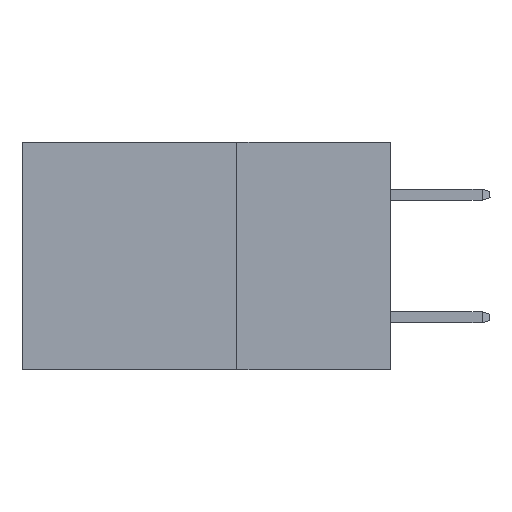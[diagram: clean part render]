
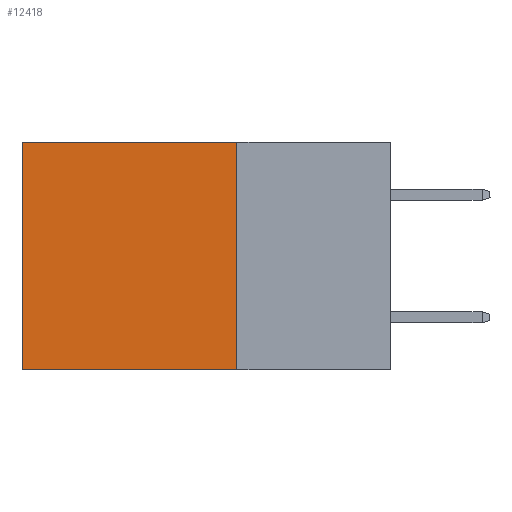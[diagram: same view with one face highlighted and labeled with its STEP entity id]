
A CAD part, left-side view. The second image highlights one B-rep face of the part: STEP entity #12418.
In plain terms, the highlighted planar face has unit normal (-1, 0, 0).
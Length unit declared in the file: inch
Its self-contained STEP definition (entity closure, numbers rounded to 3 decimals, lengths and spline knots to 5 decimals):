
#120 = ORIENTED_EDGE ( 'NONE', *, *, #13641, .F. ) ;
#557 = EDGE_CURVE ( 'NONE', #9670, #3187, #7777, .T. ) ;
#871 = EDGE_CURVE ( 'NONE', #7259, #7469, #4537, .T. ) ;
#1874 = FACE_OUTER_BOUND ( 'NONE', #2642, .T. ) ;
#1922 = CARTESIAN_POINT ( 'NONE',  ( 0.2875, 0.25, -0.37 ) ) ;
#2107 = ORIENTED_EDGE ( 'NONE', *, *, #6444, .T. ) ;
#2642 = EDGE_LOOP ( 'NONE', ( #2107, #12900, #120, #6379 ) ) ;
#2757 = DIRECTION ( 'NONE',  ( 0., 1., 0. ) ) ;
#3071 = DIRECTION ( 'NONE',  ( 0., 0., -1. ) ) ;
#3072 = VECTOR ( 'NONE', #13787, 39.37008 ) ;
#3149 = CARTESIAN_POINT ( 'NONE',  ( 0.2875, 0.6, 0. ) ) ;
#3170 = CARTESIAN_POINT ( 'NONE',  ( 0.2875, 0.25, 0. ) ) ;
#3187 = VERTEX_POINT ( 'NONE', #12374 ) ;
#3828 = VECTOR ( 'NONE', #9761, 39.37008 ) ;
#4186 = VECTOR ( 'NONE', #2757, 39.37008 ) ;
#4537 = LINE ( 'NONE', #3170, #4186 ) ;
#4897 = DIRECTION ( 'NONE',  ( 1., 0., 0. ) ) ;
#5586 = CARTESIAN_POINT ( 'NONE',  ( 0.2875, 0.25, 0. ) ) ;
#5957 = LINE ( 'NONE', #5586, #3072 ) ;
#6084 = CARTESIAN_POINT ( 'NONE',  ( 0.2875, 0.25, -0.37 ) ) ;
#6278 = VECTOR ( 'NONE', #3071, 39.37008 ) ;
#6379 = ORIENTED_EDGE ( 'NONE', *, *, #871, .T. ) ;
#6444 = EDGE_CURVE ( 'NONE', #7469, #3187, #6798, .T. ) ;
#6798 = LINE ( 'NONE', #11131, #6278 ) ;
#7259 = VERTEX_POINT ( 'NONE', #13554 ) ;
#7469 = VERTEX_POINT ( 'NONE', #3149 ) ;
#7777 = LINE ( 'NONE', #6084, #3828 ) ;
#9514 = PLANE ( 'NONE',  #9936 ) ;
#9670 = VERTEX_POINT ( 'NONE', #1922 ) ;
#9761 = DIRECTION ( 'NONE',  ( 0., 1., 0. ) ) ;
#9936 = AXIS2_PLACEMENT_3D ( 'NONE', #11616, #4897, #14061 ) ;
#11131 = CARTESIAN_POINT ( 'NONE',  ( 0.2875, 0.6, 0. ) ) ;
#11616 = CARTESIAN_POINT ( 'NONE',  ( 0.2875, 0.25, 0. ) ) ;
#12374 = CARTESIAN_POINT ( 'NONE',  ( 0.2875, 0.6, -0.37 ) ) ;
#12418 = ADVANCED_FACE ( 'NONE', ( #1874 ), #9514, .F. ) ;
#12900 = ORIENTED_EDGE ( 'NONE', *, *, #557, .F. ) ;
#13554 = CARTESIAN_POINT ( 'NONE',  ( 0.2875, 0.25, 0. ) ) ;
#13641 = EDGE_CURVE ( 'NONE', #7259, #9670, #5957, .T. ) ;
#13787 = DIRECTION ( 'NONE',  ( 0., 0., -1. ) ) ;
#14061 = DIRECTION ( 'NONE',  ( 0., 0., -1. ) ) ;
